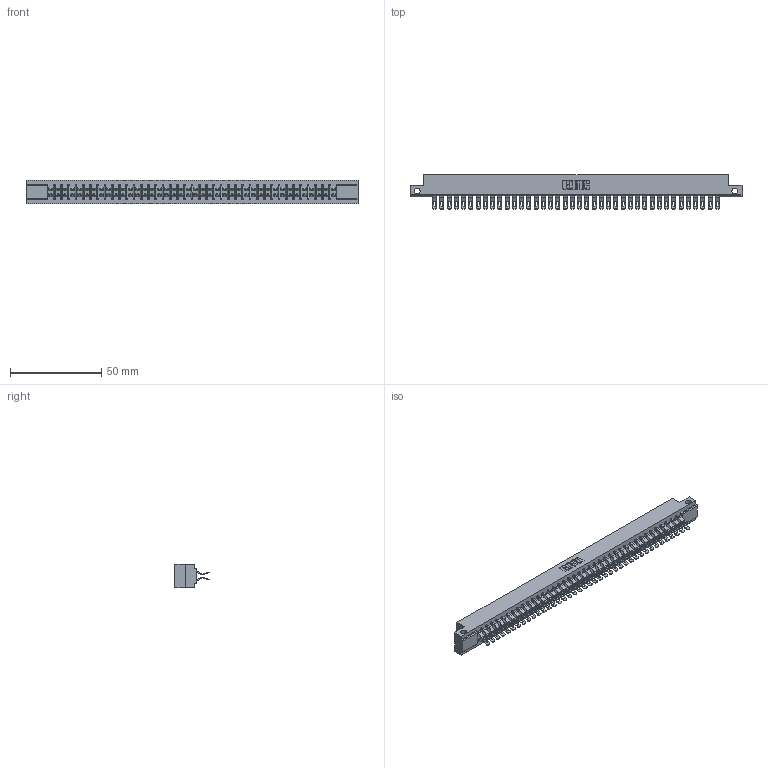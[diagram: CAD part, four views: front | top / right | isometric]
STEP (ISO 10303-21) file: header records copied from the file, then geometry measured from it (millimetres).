
FILE_DESCRIPTION (( 'STEP AP203' ), '1' );
FILE_NAME ('307-080-555-212.STEP', '2019-09-07T00:00:43', ( '' ), ( '' ), 'SwSTEP 2.0', 'SolidWorks 2016', '' );
FILE_SCHEMA (( 'CONFIG_CONTROL_DESIGN' ));
Length unit declared in the file: inch
Products named in the file (3): 307-080-555-212; 307-290-001_555; 307 Part_.128 Dia Side Mounting Holes
Assembly tree (81 placements, depth 2):
  307-080-555-212
    307 Part_.128 Dia Side Mounting Holes
    307-290-001_555  x80
Bounding box: 181.51 x 18.75 x 12.7 mm (x, y, z)
Volume: 19383.3 mm3; surface area: 24984.7 mm2
Topology: 81 solids, 81 shells, 5039 faces, 14803 edges, 9650 vertices
Faces by surface type: plane 2790, cylinder 2167, sphere 82
Entity records: 36357 total; most frequent: CARTESIAN_POINT 5952, ORIENTED_EDGE 5900, DIRECTION 5838, EDGE_CURVE 2950, VECTOR 2250, LINE 2250, VERTEX_POINT 1908, AXIS2_PLACEMENT_3D 1794
